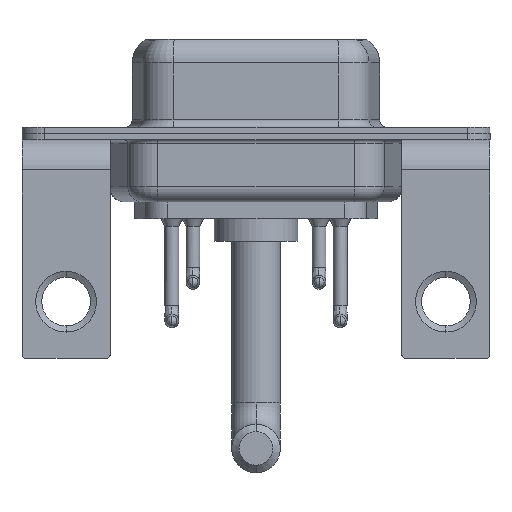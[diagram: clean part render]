
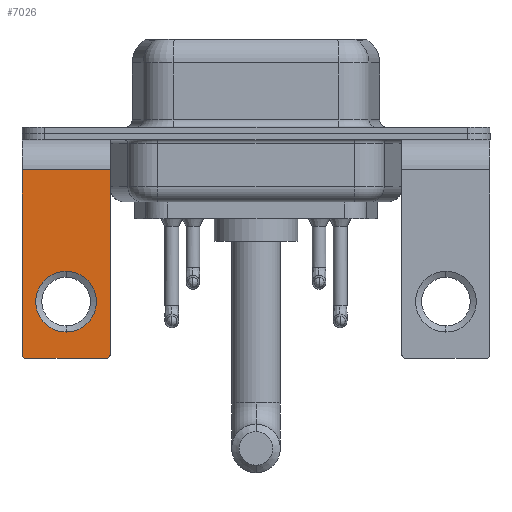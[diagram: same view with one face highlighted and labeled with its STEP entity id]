
A CAD part, front view. The second image highlights one B-rep face of the part: STEP entity #7026.
In plain terms, the highlighted planar face has unit normal (0, -1, 0).
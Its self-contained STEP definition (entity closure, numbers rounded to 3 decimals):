
#152 = AXIS2_PLACEMENT_3D ( 'NONE', #10936, #16206, #4355 ) ;
#246 = VERTEX_POINT ( 'NONE', #15279 ) ;
#505 = ORIENTED_EDGE ( 'NONE', *, *, #7980, .T. ) ;
#1158 = ORIENTED_EDGE ( 'NONE', *, *, #14158, .T. ) ;
#1172 = DIRECTION ( 'NONE',  ( 0., 1., 0. ) ) ;
#1612 = CARTESIAN_POINT ( 'NONE',  ( 0., -6.25, -9.07 ) ) ;
#1900 = DIRECTION ( 'NONE',  ( -1., 0., 0. ) ) ;
#2049 = CIRCLE ( 'NONE', #15580, 2. ) ;
#2209 = VERTEX_POINT ( 'NONE', #7342 ) ;
#2421 = DIRECTION ( 'NONE',  ( 0., -1., 0. ) ) ;
#2469 = DIRECTION ( 'NONE',  ( -1., 0., 0. ) ) ;
#2648 = CARTESIAN_POINT ( 'NONE',  ( 0., -6.25, -13.07 ) ) ;
#2653 = DIRECTION ( 'NONE',  ( 0., 1., 0. ) ) ;
#2734 = CARTESIAN_POINT ( 'NONE',  ( 2.9, -6.25, -2.4 ) ) ;
#4137 = EDGE_CURVE ( 'NONE', #2209, #246, #12503, .T. ) ;
#4240 = CIRCLE ( 'NONE', #6464, 2. ) ;
#4355 = DIRECTION ( 'NONE',  ( 0., 0., 1. ) ) ;
#5152 = CARTESIAN_POINT ( 'NONE',  ( 2.9, -6.25, -2.4 ) ) ;
#5238 = DIRECTION ( 'NONE',  ( 0., 1., 0. ) ) ;
#5356 = ORIENTED_EDGE ( 'NONE', *, *, #12418, .T. ) ;
#5879 = LINE ( 'NONE', #13574, #12319 ) ;
#5951 = VECTOR ( 'NONE', #6775, 1000. ) ;
#6037 = ORIENTED_EDGE ( 'NONE', *, *, #4137, .T. ) ;
#6095 = EDGE_LOOP ( 'NONE', ( #9322, #10152, #6127, #6037, #16631, #1158 ) ) ;
#6127 = ORIENTED_EDGE ( 'NONE', *, *, #15210, .F. ) ;
#6238 = CARTESIAN_POINT ( 'NONE',  ( -2.9, -6.25, -14.55 ) ) ;
#6348 = DIRECTION ( 'NONE',  ( 0., 0., 1. ) ) ;
#6464 = AXIS2_PLACEMENT_3D ( 'NONE', #13205, #1172, #10433 ) ;
#6570 = VERTEX_POINT ( 'NONE', #6238 ) ;
#6775 = DIRECTION ( 'NONE',  ( 0., 0., -1. ) ) ;
#6928 = CARTESIAN_POINT ( 'NONE',  ( -2.65, -6.25, -14.8 ) ) ;
#6999 = DIRECTION ( 'NONE',  ( 0., 0., -1. ) ) ;
#7026 = ADVANCED_FACE ( 'NONE', ( #16916, #14330 ), #10507, .F. ) ;
#7334 = AXIS2_PLACEMENT_3D ( 'NONE', #5152, #5238, #14068 ) ;
#7342 = CARTESIAN_POINT ( 'NONE',  ( 2.65, -6.25, -14.8 ) ) ;
#7523 = AXIS2_PLACEMENT_3D ( 'NONE', #15842, #2421, #6348 ) ;
#7955 = LINE ( 'NONE', #2734, #10327 ) ;
#7956 = DIRECTION ( 'NONE',  ( 0., 0., 1. ) ) ;
#7980 = EDGE_CURVE ( 'NONE', #11974, #8724, #2049, .T. ) ;
#8035 = CARTESIAN_POINT ( 'NONE',  ( 2.9, -6.25, -2.4 ) ) ;
#8048 = VERTEX_POINT ( 'NONE', #8035 ) ;
#8307 = CARTESIAN_POINT ( 'NONE',  ( 2.9, -6.25, -14.8 ) ) ;
#8568 = LINE ( 'NONE', #8307, #14505 ) ;
#8724 = VERTEX_POINT ( 'NONE', #2648 ) ;
#9322 = ORIENTED_EDGE ( 'NONE', *, *, #9694, .T. ) ;
#9694 = EDGE_CURVE ( 'NONE', #13773, #6570, #13785, .T. ) ;
#10152 = ORIENTED_EDGE ( 'NONE', *, *, #12829, .T. ) ;
#10327 = VECTOR ( 'NONE', #2469, 1000. ) ;
#10433 = DIRECTION ( 'NONE',  ( 0., 0., 1. ) ) ;
#10507 = PLANE ( 'NONE',  #7334 ) ;
#10936 = CARTESIAN_POINT ( 'NONE',  ( -2.65, -6.25, -14.55 ) ) ;
#11974 = VERTEX_POINT ( 'NONE', #1612 ) ;
#12319 = VECTOR ( 'NONE', #6999, 1000. ) ;
#12418 = EDGE_CURVE ( 'NONE', #8724, #11974, #4240, .T. ) ;
#12503 = CIRCLE ( 'NONE', #7523, 0.25 ) ;
#12829 = EDGE_CURVE ( 'NONE', #6570, #13735, #14478, .T. ) ;
#13205 = CARTESIAN_POINT ( 'NONE',  ( 0., -6.25, -11.07 ) ) ;
#13574 = CARTESIAN_POINT ( 'NONE',  ( 2.9, -6.25, -2.4 ) ) ;
#13735 = VERTEX_POINT ( 'NONE', #6928 ) ;
#13773 = VERTEX_POINT ( 'NONE', #16254 ) ;
#13785 = LINE ( 'NONE', #16097, #5951 ) ;
#14068 = DIRECTION ( 'NONE',  ( 0., 0., 1. ) ) ;
#14158 = EDGE_CURVE ( 'NONE', #8048, #13773, #7955, .T. ) ;
#14330 = FACE_OUTER_BOUND ( 'NONE', #6095, .T. ) ;
#14478 = CIRCLE ( 'NONE', #152, 0.25 ) ;
#14505 = VECTOR ( 'NONE', #1900, 1000. ) ;
#15210 = EDGE_CURVE ( 'NONE', #2209, #13735, #8568, .T. ) ;
#15279 = CARTESIAN_POINT ( 'NONE',  ( 2.9, -6.25, -14.55 ) ) ;
#15480 = EDGE_LOOP ( 'NONE', ( #5356, #505 ) ) ;
#15580 = AXIS2_PLACEMENT_3D ( 'NONE', #15808, #2653, #7956 ) ;
#15706 = EDGE_CURVE ( 'NONE', #8048, #246, #5879, .T. ) ;
#15808 = CARTESIAN_POINT ( 'NONE',  ( 0., -6.25, -11.07 ) ) ;
#15842 = CARTESIAN_POINT ( 'NONE',  ( 2.65, -6.25, -14.55 ) ) ;
#16097 = CARTESIAN_POINT ( 'NONE',  ( -2.9, -6.25, -2.4 ) ) ;
#16206 = DIRECTION ( 'NONE',  ( 0., -1., 0. ) ) ;
#16254 = CARTESIAN_POINT ( 'NONE',  ( -2.9, -6.25, -2.4 ) ) ;
#16631 = ORIENTED_EDGE ( 'NONE', *, *, #15706, .F. ) ;
#16916 = FACE_BOUND ( 'NONE', #15480, .T. ) ;
